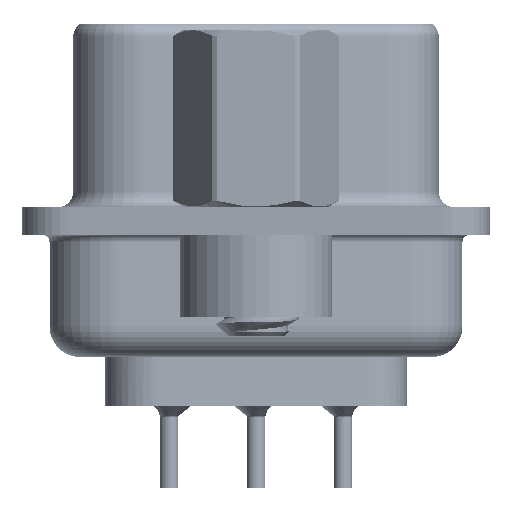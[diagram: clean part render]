
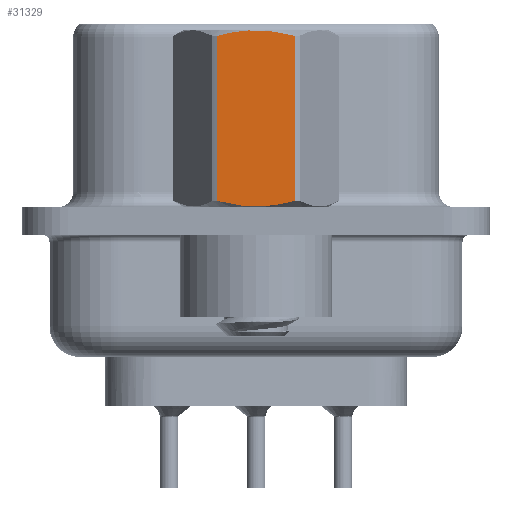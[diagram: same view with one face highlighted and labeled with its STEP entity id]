
A CAD part, left-side view. The second image highlights one B-rep face of the part: STEP entity #31329.
In plain terms, the highlighted planar face has unit normal (-1, 0, 0).
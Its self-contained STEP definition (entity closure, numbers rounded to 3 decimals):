
#485 = LINE ( 'NONE', #17095, #39956 ) ;
#2861 = CARTESIAN_POINT ( 'NONE',  ( -2.381, 0.853, 0.549 ) ) ;
#3040 = CARTESIAN_POINT ( 'NONE',  ( -2.381, -1.273, 6.048 ) ) ;
#3148 = B_SPLINE_CURVE_WITH_KNOTS ( 'NONE', 3,
 ( #3040, #37196, #15392, #24800, #6162, #27954, #9290, #31100, #12409, #34204 ),
 .UNSPECIFIED., .F., .F.,
 ( 4, 2, 2, 2, 4 ),
 ( 0.001, 0.002, 0.002, 0.003, 0.004 ),
 .UNSPECIFIED. ) ;
#5792 = EDGE_CURVE ( 'NONE', #22352, #31888, #3148, .T. ) ;
#6162 = CARTESIAN_POINT ( 'NONE',  ( -2.381, -0.215, 6.232 ) ) ;
#7684 = CARTESIAN_POINT ( 'NONE',  ( -2.381, 1.273, 0.652 ) ) ;
#7789 = AXIS2_PLACEMENT_3D ( 'NONE', #20369, #11133, #32930 ) ;
#8006 = PLANE ( 'NONE',  #7789 ) ;
#9115 = CARTESIAN_POINT ( 'NONE',  ( -2.381, 1.273, 0.652 ) ) ;
#9290 = CARTESIAN_POINT ( 'NONE',  ( -2.381, 0.428, 6.215 ) ) ;
#10052 = FACE_OUTER_BOUND ( 'NONE', #33254, .T. ) ;
#10246 = CARTESIAN_POINT ( 'NONE',  ( -2.381, -1.273, 0.652 ) ) ;
#10800 = LINE ( 'NONE', #24407, #26427 ) ;
#11082 = CARTESIAN_POINT ( 'NONE',  ( -2.381, 1.273, 6.048 ) ) ;
#11133 = DIRECTION ( 'NONE',  ( -1., 0., 0. ) ) ;
#12231 = CARTESIAN_POINT ( 'NONE',  ( -2.381, 0.215, 0.468 ) ) ;
#12409 = CARTESIAN_POINT ( 'NONE',  ( -2.381, 1.065, 6.104 ) ) ;
#12545 = EDGE_CURVE ( 'NONE', #29622, #21974, #26317, .T. ) ;
#15341 = CARTESIAN_POINT ( 'NONE',  ( -2.381, -0.432, 0.485 ) ) ;
#15392 = CARTESIAN_POINT ( 'NONE',  ( -2.381, -0.858, 6.15 ) ) ;
#17095 = CARTESIAN_POINT ( 'NONE',  ( -2.381, 1.273, 3.792 ) ) ;
#18464 = CARTESIAN_POINT ( 'NONE',  ( -2.381, -1.066, 0.596 ) ) ;
#20369 = CARTESIAN_POINT ( 'NONE',  ( -2.381, 1.375, -3.75 ) ) ;
#21473 = CARTESIAN_POINT ( 'NONE',  ( -2.381, 1.065, 0.596 ) ) ;
#21974 = VERTEX_POINT ( 'NONE', #10246 ) ;
#22352 = VERTEX_POINT ( 'NONE', #34211 ) ;
#23503 = DIRECTION ( 'NONE',  ( 0., 0., -1. ) ) ;
#24407 = CARTESIAN_POINT ( 'NONE',  ( -2.381, -1.273, 3.792 ) ) ;
#24800 = CARTESIAN_POINT ( 'NONE',  ( -2.381, -0.432, 6.215 ) ) ;
#26317 = B_SPLINE_CURVE_WITH_KNOTS ( 'NONE', 3,
 ( #9115, #21473, #2861, #30925, #12231, #34027, #15341, #37150, #18464, #40251 ),
 .UNSPECIFIED., .F., .F.,
 ( 4, 2, 2, 2, 4 ),
 ( 0.003, 0.003, 0.004, 0.004, 0.005 ),
 .UNSPECIFIED. ) ;
#26426 = ORIENTED_EDGE ( 'NONE', *, *, #12545, .T. ) ;
#26427 = VECTOR ( 'NONE', #33821, 1000. ) ;
#26911 = EDGE_CURVE ( 'NONE', #21974, #22352, #10800, .T. ) ;
#27954 = CARTESIAN_POINT ( 'NONE',  ( -2.381, 0.215, 6.232 ) ) ;
#28032 = ORIENTED_EDGE ( 'NONE', *, *, #5792, .T. ) ;
#28980 = EDGE_CURVE ( 'NONE', #31888, #29622, #485, .T. ) ;
#29622 = VERTEX_POINT ( 'NONE', #7684 ) ;
#30925 = CARTESIAN_POINT ( 'NONE',  ( -2.381, 0.428, 0.485 ) ) ;
#31100 = CARTESIAN_POINT ( 'NONE',  ( -2.381, 0.853, 6.151 ) ) ;
#31329 = ADVANCED_FACE ( 'NONE', ( #10052 ), #8006, .T. ) ;
#31888 = VERTEX_POINT ( 'NONE', #11082 ) ;
#32930 = DIRECTION ( 'NONE',  ( 0., -1., 0. ) ) ;
#33254 = EDGE_LOOP ( 'NONE', ( #26426, #33337, #28032, #37480 ) ) ;
#33337 = ORIENTED_EDGE ( 'NONE', *, *, #26911, .T. ) ;
#33821 = DIRECTION ( 'NONE',  ( 0., 0., 1. ) ) ;
#34027 = CARTESIAN_POINT ( 'NONE',  ( -2.381, -0.215, 0.468 ) ) ;
#34204 = CARTESIAN_POINT ( 'NONE',  ( -2.381, 1.273, 6.048 ) ) ;
#34211 = CARTESIAN_POINT ( 'NONE',  ( -2.381, -1.273, 6.048 ) ) ;
#37150 = CARTESIAN_POINT ( 'NONE',  ( -2.381, -0.858, 0.55 ) ) ;
#37196 = CARTESIAN_POINT ( 'NONE',  ( -2.381, -1.066, 6.104 ) ) ;
#37480 = ORIENTED_EDGE ( 'NONE', *, *, #28980, .T. ) ;
#39956 = VECTOR ( 'NONE', #23503, 1000. ) ;
#40251 = CARTESIAN_POINT ( 'NONE',  ( -2.381, -1.273, 0.652 ) ) ;
